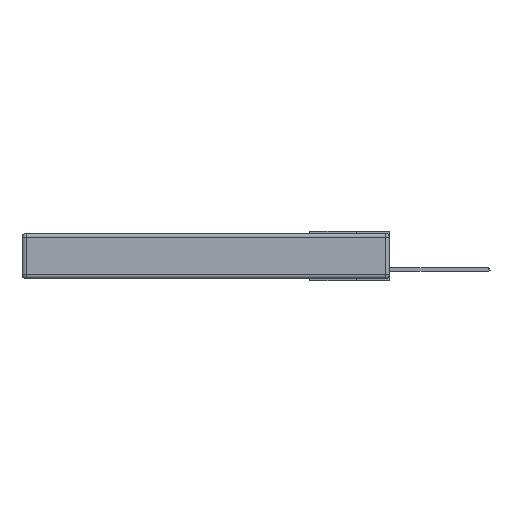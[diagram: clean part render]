
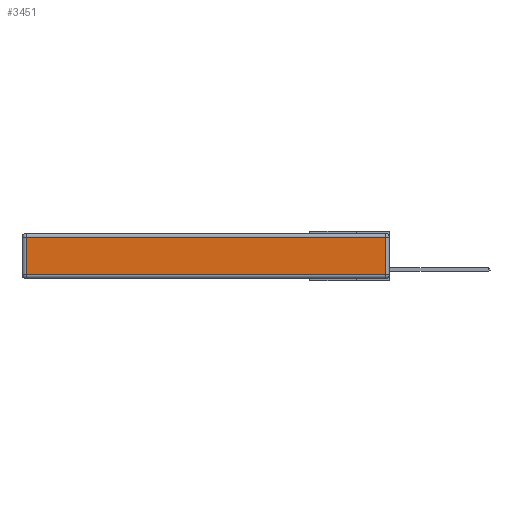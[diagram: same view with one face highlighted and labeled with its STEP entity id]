
A CAD part, left-side view. The second image highlights one B-rep face of the part: STEP entity #3451.
In plain terms, the highlighted planar face has unit normal (-1, 0, 0).
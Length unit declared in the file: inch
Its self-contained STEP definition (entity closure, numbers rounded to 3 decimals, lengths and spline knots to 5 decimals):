
#1217 = CARTESIAN_POINT ( 'NONE',  ( 0., 0.03, -0.03 ) ) ;
#2397 = DIRECTION ( 'NONE',  ( -1., 0., 0. ) ) ;
#2643 = ORIENTED_EDGE ( 'NONE', *, *, #5356, .T. ) ;
#2921 = VECTOR ( 'NONE', #7755, 39.37008 ) ;
#3005 = ORIENTED_EDGE ( 'NONE', *, *, #15170, .T. ) ;
#3204 = VECTOR ( 'NONE', #6154, 39.37008 ) ;
#3451 = ADVANCED_FACE ( 'NONE', ( #3455 ), #13118, .T. ) ;
#3455 = FACE_OUTER_BOUND ( 'NONE', #11604, .T. ) ;
#3624 = CARTESIAN_POINT ( 'NONE',  ( 0., 2.72, -0.03 ) ) ;
#4476 = LINE ( 'NONE', #16773, #3204 ) ;
#5356 = EDGE_CURVE ( 'NONE', #8658, #8893, #4476, .T. ) ;
#6154 = DIRECTION ( 'NONE',  ( 0., 0., 1. ) ) ;
#6198 = AXIS2_PLACEMENT_3D ( 'NONE', #15843, #2397, #9172 ) ;
#6368 = ORIENTED_EDGE ( 'NONE', *, *, #16729, .T. ) ;
#7695 = CARTESIAN_POINT ( 'NONE',  ( 0., 0., -0.313 ) ) ;
#7755 = DIRECTION ( 'NONE',  ( 0., 0., -1. ) ) ;
#7798 = DIRECTION ( 'NONE',  ( 0., -1., 0. ) ) ;
#7802 = VECTOR ( 'NONE', #7798, 39.37008 ) ;
#7810 = CARTESIAN_POINT ( 'NONE',  ( 0., 2.72, -0.343 ) ) ;
#8635 = DIRECTION ( 'NONE',  ( 0., 1., 0. ) ) ;
#8658 = VERTEX_POINT ( 'NONE', #14435 ) ;
#8823 = LINE ( 'NONE', #7810, #2921 ) ;
#8889 = EDGE_CURVE ( 'NONE', #9115, #8658, #14099, .T. ) ;
#8893 = VERTEX_POINT ( 'NONE', #1217 ) ;
#9115 = VERTEX_POINT ( 'NONE', #12932 ) ;
#9172 = DIRECTION ( 'NONE',  ( 0., 0., 1. ) ) ;
#9801 = VERTEX_POINT ( 'NONE', #3624 ) ;
#9960 = ORIENTED_EDGE ( 'NONE', *, *, #8889, .T. ) ;
#10200 = LINE ( 'NONE', #16576, #14163 ) ;
#11604 = EDGE_LOOP ( 'NONE', ( #9960, #2643, #3005, #6368 ) ) ;
#12932 = CARTESIAN_POINT ( 'NONE',  ( 0., 2.72, -0.313 ) ) ;
#13118 = PLANE ( 'NONE',  #6198 ) ;
#14099 = LINE ( 'NONE', #7695, #7802 ) ;
#14163 = VECTOR ( 'NONE', #8635, 39.37008 ) ;
#14435 = CARTESIAN_POINT ( 'NONE',  ( 0., 0.03, -0.313 ) ) ;
#15170 = EDGE_CURVE ( 'NONE', #8893, #9801, #10200, .T. ) ;
#15843 = CARTESIAN_POINT ( 'NONE',  ( 0., 0., -0.343 ) ) ;
#16576 = CARTESIAN_POINT ( 'NONE',  ( 0., 2.75, -0.03 ) ) ;
#16729 = EDGE_CURVE ( 'NONE', #9801, #9115, #8823, .T. ) ;
#16773 = CARTESIAN_POINT ( 'NONE',  ( 0., 0.03, -0.343 ) ) ;
